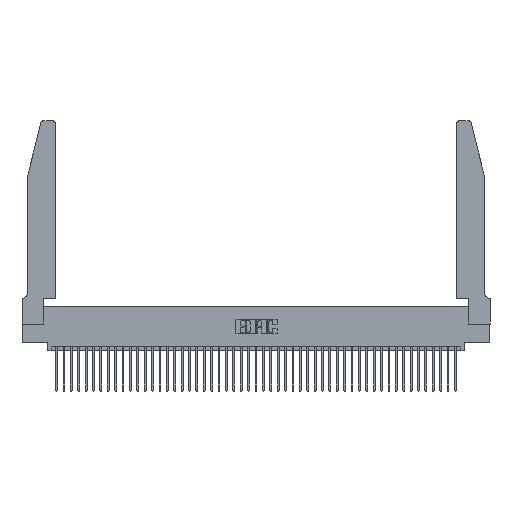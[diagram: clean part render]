
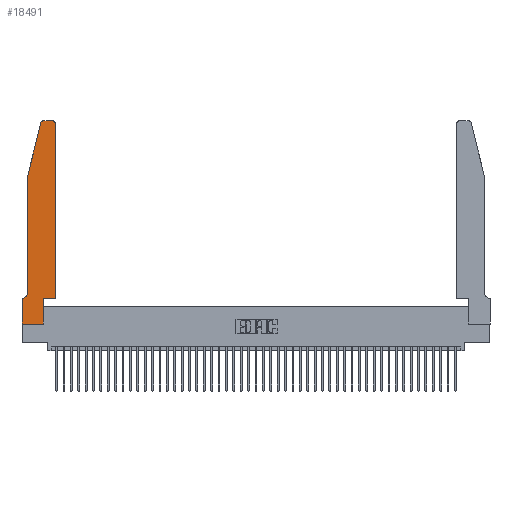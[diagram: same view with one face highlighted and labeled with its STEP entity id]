
A CAD part, top view. The second image highlights one B-rep face of the part: STEP entity #18491.
In plain terms, the highlighted planar face has unit normal (0, 0, 1).
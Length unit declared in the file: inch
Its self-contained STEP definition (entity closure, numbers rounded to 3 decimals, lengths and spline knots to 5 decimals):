
#157 = EDGE_CURVE ( 'NONE', #35747, #11408, #31950, .T. ) ;
#503 = VECTOR ( 'NONE', #8709, 39.37008 ) ;
#1093 = VERTEX_POINT ( 'NONE', #31513 ) ;
#3391 = ORIENTED_EDGE ( 'NONE', *, *, #44566, .T. ) ;
#3592 = CARTESIAN_POINT ( 'NONE',  ( 0.284, 2.75, 0.37 ) ) ;
#3837 = CARTESIAN_POINT ( 'NONE',  ( 0.0755, 0.35, 0.37 ) ) ;
#4013 = EDGE_CURVE ( 'NONE', #29761, #40247, #41669, .T. ) ;
#5522 = CARTESIAN_POINT ( 'NONE',  ( 0.284, 2.72, 0.37 ) ) ;
#5643 = CIRCLE ( 'NONE', #5774, 0.07 ) ;
#5774 = AXIS2_PLACEMENT_3D ( 'NONE', #30005, #8603, #33592 ) ;
#6351 = AXIS2_PLACEMENT_3D ( 'NONE', #5522, #30576, #9198 ) ;
#6449 = CARTESIAN_POINT ( 'NONE',  ( 0., 0., 0.37 ) ) ;
#6883 = PLANE ( 'NONE',  #40117 ) ;
#7313 = EDGE_CURVE ( 'NONE', #40247, #9904, #34820, .T. ) ;
#8393 = CARTESIAN_POINT ( 'NONE',  ( 0.2865, 0.35, 0.37 ) ) ;
#8603 = DIRECTION ( 'NONE',  ( 0., 0., -1. ) ) ;
#8709 = DIRECTION ( 'NONE',  ( 0., 1., 0. ) ) ;
#8734 = VERTEX_POINT ( 'NONE', #17414 ) ;
#9198 = DIRECTION ( 'NONE',  ( 1., 0., 0. ) ) ;
#9624 = CARTESIAN_POINT ( 'NONE',  ( 0.4505, 2.72, 0.37 ) ) ;
#9904 = VERTEX_POINT ( 'NONE', #9624 ) ;
#10081 = DIRECTION ( 'NONE',  ( 1., 0., 0. ) ) ;
#10355 = CARTESIAN_POINT ( 'NONE',  ( 0.4505, 0.35, 0.37 ) ) ;
#11408 = VERTEX_POINT ( 'NONE', #3592 ) ;
#11412 = CARTESIAN_POINT ( 'NONE',  ( 0.25487, 2.72718, 0.37 ) ) ;
#11656 = VERTEX_POINT ( 'NONE', #32598 ) ;
#11711 = ORIENTED_EDGE ( 'NONE', *, *, #21572, .T. ) ;
#12482 = ORIENTED_EDGE ( 'NONE', *, *, #4013, .T. ) ;
#12609 = ORIENTED_EDGE ( 'NONE', *, *, #157, .T. ) ;
#13191 = VECTOR ( 'NONE', #15550, 39.37008 ) ;
#14139 = DIRECTION ( 'NONE',  ( 1., 0., 0. ) ) ;
#14227 = EDGE_CURVE ( 'NONE', #1093, #36775, #35682, .T. ) ;
#14243 = VECTOR ( 'NONE', #10081, 39.37008 ) ;
#14869 = CARTESIAN_POINT ( 'NONE',  ( 0.0755, 0.42, 0.37 ) ) ;
#15038 = ORIENTED_EDGE ( 'NONE', *, *, #31545, .T. ) ;
#15208 = VERTEX_POINT ( 'NONE', #14869 ) ;
#15380 = ORIENTED_EDGE ( 'NONE', *, *, #20683, .T. ) ;
#15550 = DIRECTION ( 'NONE',  ( -0.239, -0.971, 0. ) ) ;
#16040 = ORIENTED_EDGE ( 'NONE', *, *, #30100, .T. ) ;
#17062 = CARTESIAN_POINT ( 'NONE',  ( 0.0055, 0.35, 0.37 ) ) ;
#17414 = CARTESIAN_POINT ( 'NONE',  ( 0.2865, 0., 0.37 ) ) ;
#17770 = LINE ( 'NONE', #36754, #43866 ) ;
#18491 = ADVANCED_FACE ( 'NONE', ( #23090 ), #6883, .T. ) ;
#18895 = DIRECTION ( 'NONE',  ( 0., 0., 1. ) ) ;
#19029 = DIRECTION ( 'NONE',  ( 0., -1., 0. ) ) ;
#19073 = CIRCLE ( 'NONE', #6351, 0.03 ) ;
#19824 = DIRECTION ( 'NONE',  ( 1., 0., 0. ) ) ;
#20683 = EDGE_CURVE ( 'NONE', #36775, #8734, #23666, .T. ) ;
#21572 = EDGE_CURVE ( 'NONE', #15208, #31174, #5643, .T. ) ;
#21623 = DIRECTION ( 'NONE',  ( 0., -1., 0. ) ) ;
#22125 = EDGE_CURVE ( 'NONE', #8734, #29761, #38638, .T. ) ;
#22462 = VECTOR ( 'NONE', #33483, 39.37008 ) ;
#23090 = FACE_OUTER_BOUND ( 'NONE', #31144, .T. ) ;
#23430 = VECTOR ( 'NONE', #32554, 39.37008 ) ;
#23666 = LINE ( 'NONE', #6449, #14243 ) ;
#23734 = LINE ( 'NONE', #33292, #13191 ) ;
#24779 = ORIENTED_EDGE ( 'NONE', *, *, #45658, .T. ) ;
#26333 = CARTESIAN_POINT ( 'NONE',  ( 0., 0., 0.37 ) ) ;
#26719 = ORIENTED_EDGE ( 'NONE', *, *, #7313, .T. ) ;
#26850 = ORIENTED_EDGE ( 'NONE', *, *, #22125, .T. ) ;
#29588 = LINE ( 'NONE', #3837, #23430 ) ;
#29761 = VERTEX_POINT ( 'NONE', #41386 ) ;
#30005 = CARTESIAN_POINT ( 'NONE',  ( 0.0055, 0.42, 0.37 ) ) ;
#30100 = EDGE_CURVE ( 'NONE', #31174, #1093, #29588, .T. ) ;
#30576 = DIRECTION ( 'NONE',  ( 0., 0., 1. ) ) ;
#31144 = EDGE_LOOP ( 'NONE', ( #12609, #43110, #24779, #15038, #11711, #16040, #41043, #15380, #26850, #12482, #26719, #3391 ) ) ;
#31174 = VERTEX_POINT ( 'NONE', #17062 ) ;
#31513 = CARTESIAN_POINT ( 'NONE',  ( 0., 0.35, 0.37 ) ) ;
#31545 = EDGE_CURVE ( 'NONE', #11656, #15208, #17770, .T. ) ;
#31886 = CARTESIAN_POINT ( 'NONE',  ( 0., 0.35, 0.37 ) ) ;
#31950 = LINE ( 'NONE', #37163, #22462 ) ;
#32259 = VECTOR ( 'NONE', #19824, 39.37008 ) ;
#32554 = DIRECTION ( 'NONE',  ( -1., 0., 0. ) ) ;
#32594 = VECTOR ( 'NONE', #41417, 39.37008 ) ;
#32598 = CARTESIAN_POINT ( 'NONE',  ( 0.0755, 2., 0.37 ) ) ;
#33292 = CARTESIAN_POINT ( 'NONE',  ( 0.0755, 2., 0.37 ) ) ;
#33483 = DIRECTION ( 'NONE',  ( -1., 0., 0. ) ) ;
#33592 = DIRECTION ( 'NONE',  ( -1., 0., 0. ) ) ;
#34820 = LINE ( 'NONE', #37865, #32594 ) ;
#35151 = CARTESIAN_POINT ( 'NONE',  ( 0.4205, 2.75, 0.37 ) ) ;
#35471 = DIRECTION ( 'NONE',  ( 0., 0., 1. ) ) ;
#35682 = LINE ( 'NONE', #39343, #43982 ) ;
#35747 = VERTEX_POINT ( 'NONE', #35151 ) ;
#36754 = CARTESIAN_POINT ( 'NONE',  ( 0.0755, 2., 0.37 ) ) ;
#36775 = VERTEX_POINT ( 'NONE', #26333 ) ;
#37163 = CARTESIAN_POINT ( 'NONE',  ( 0.2605, 2.75, 0.37 ) ) ;
#37865 = CARTESIAN_POINT ( 'NONE',  ( 0.4505, 0.35, 0.37 ) ) ;
#38638 = LINE ( 'NONE', #8393, #503 ) ;
#39157 = VERTEX_POINT ( 'NONE', #11412 ) ;
#39293 = AXIS2_PLACEMENT_3D ( 'NONE', #40176, #18895, #43745 ) ;
#39343 = CARTESIAN_POINT ( 'NONE',  ( 0., 0., 0.37 ) ) ;
#39997 = CIRCLE ( 'NONE', #39293, 0.03 ) ;
#40117 = AXIS2_PLACEMENT_3D ( 'NONE', #31886, #35471, #14139 ) ;
#40176 = CARTESIAN_POINT ( 'NONE',  ( 0.4205, 2.72, 0.37 ) ) ;
#40247 = VERTEX_POINT ( 'NONE', #10355 ) ;
#41043 = ORIENTED_EDGE ( 'NONE', *, *, #14227, .T. ) ;
#41108 = CARTESIAN_POINT ( 'NONE',  ( 0.4505, 0.35, 0.37 ) ) ;
#41386 = CARTESIAN_POINT ( 'NONE',  ( 0.2865, 0.35, 0.37 ) ) ;
#41417 = DIRECTION ( 'NONE',  ( 0., 1., 0. ) ) ;
#41669 = LINE ( 'NONE', #41108, #32259 ) ;
#42330 = EDGE_CURVE ( 'NONE', #11408, #39157, #19073, .T. ) ;
#43110 = ORIENTED_EDGE ( 'NONE', *, *, #42330, .T. ) ;
#43745 = DIRECTION ( 'NONE',  ( 1., 0., 0. ) ) ;
#43866 = VECTOR ( 'NONE', #19029, 39.37008 ) ;
#43982 = VECTOR ( 'NONE', #21623, 39.37008 ) ;
#44566 = EDGE_CURVE ( 'NONE', #9904, #35747, #39997, .T. ) ;
#45658 = EDGE_CURVE ( 'NONE', #39157, #11656, #23734, .T. ) ;
